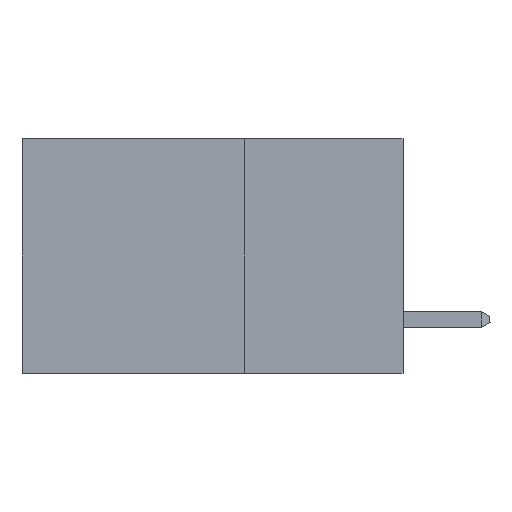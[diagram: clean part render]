
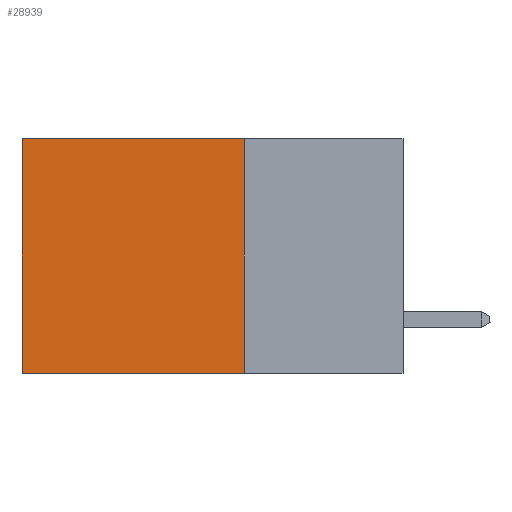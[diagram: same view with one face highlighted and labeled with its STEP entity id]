
A CAD part, left-side view. The second image highlights one B-rep face of the part: STEP entity #28939.
In plain terms, the highlighted planar face has unit normal (-1, 0, 0).
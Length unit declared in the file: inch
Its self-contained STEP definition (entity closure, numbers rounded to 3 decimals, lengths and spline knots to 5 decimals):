
#2634 = VECTOR ( 'NONE', #6581, 39.37008 ) ;
#3303 = ORIENTED_EDGE ( 'NONE', *, *, #19304, .T. ) ;
#4909 = LINE ( 'NONE', #5809, #2634 ) ;
#5657 = FACE_OUTER_BOUND ( 'NONE', #24304, .T. ) ;
#5809 = CARTESIAN_POINT ( 'NONE',  ( 0.2875, 0.6, 0. ) ) ;
#6581 = DIRECTION ( 'NONE',  ( 0., 0., -1. ) ) ;
#7853 = CARTESIAN_POINT ( 'NONE',  ( 0.2875, 0.25, 0. ) ) ;
#7876 = ORIENTED_EDGE ( 'NONE', *, *, #19016, .F. ) ;
#10272 = EDGE_CURVE ( 'NONE', #22304, #23804, #30280, .T. ) ;
#11799 = ORIENTED_EDGE ( 'NONE', *, *, #23182, .T. ) ;
#13109 = CARTESIAN_POINT ( 'NONE',  ( 0.2875, 0.25, 0. ) ) ;
#16515 = VECTOR ( 'NONE', #20355, 39.37008 ) ;
#17065 = VERTEX_POINT ( 'NONE', #28674 ) ;
#17514 = DIRECTION ( 'NONE',  ( 0., 0., -1. ) ) ;
#19016 = EDGE_CURVE ( 'NONE', #23804, #28006, #24420, .T. ) ;
#19254 = DIRECTION ( 'NONE',  ( 0., 1., 0. ) ) ;
#19304 = EDGE_CURVE ( 'NONE', #17065, #28006, #4909, .T. ) ;
#20099 = CARTESIAN_POINT ( 'NONE',  ( 0.2875, 0.25, 0. ) ) ;
#20196 = DIRECTION ( 'NONE',  ( 0., 0., -1. ) ) ;
#20355 = DIRECTION ( 'NONE',  ( 0., 1., 0. ) ) ;
#20423 = PLANE ( 'NONE',  #29474 ) ;
#20615 = VECTOR ( 'NONE', #19254, 39.37008 ) ;
#21569 = VECTOR ( 'NONE', #17514, 39.37008 ) ;
#22199 = LINE ( 'NONE', #7853, #16515 ) ;
#22304 = VERTEX_POINT ( 'NONE', #20099 ) ;
#23182 = EDGE_CURVE ( 'NONE', #22304, #17065, #22199, .T. ) ;
#23804 = VERTEX_POINT ( 'NONE', #31601 ) ;
#23871 = CARTESIAN_POINT ( 'NONE',  ( 0.2875, 0.25, -0.37 ) ) ;
#24304 = EDGE_LOOP ( 'NONE', ( #3303, #7876, #30672, #11799 ) ) ;
#24420 = LINE ( 'NONE', #23871, #20615 ) ;
#24552 = CARTESIAN_POINT ( 'NONE',  ( 0.2875, 0.25, 0. ) ) ;
#27339 = CARTESIAN_POINT ( 'NONE',  ( 0.2875, 0.6, -0.37 ) ) ;
#27866 = DIRECTION ( 'NONE',  ( 1., 0., 0. ) ) ;
#28006 = VERTEX_POINT ( 'NONE', #27339 ) ;
#28674 = CARTESIAN_POINT ( 'NONE',  ( 0.2875, 0.6, 0. ) ) ;
#28939 = ADVANCED_FACE ( 'NONE', ( #5657 ), #20423, .F. ) ;
#29474 = AXIS2_PLACEMENT_3D ( 'NONE', #13109, #27866, #20196 ) ;
#30280 = LINE ( 'NONE', #24552, #21569 ) ;
#30672 = ORIENTED_EDGE ( 'NONE', *, *, #10272, .F. ) ;
#31601 = CARTESIAN_POINT ( 'NONE',  ( 0.2875, 0.25, -0.37 ) ) ;
